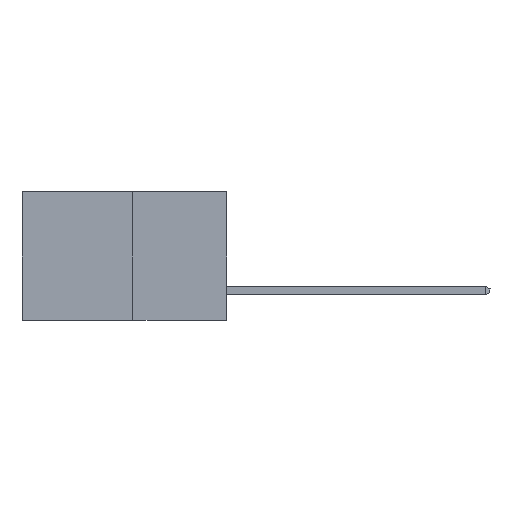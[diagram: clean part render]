
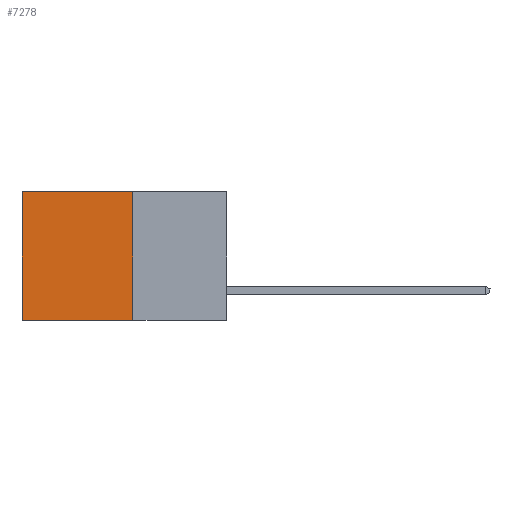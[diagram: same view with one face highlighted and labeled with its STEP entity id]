
A CAD part, left-side view. The second image highlights one B-rep face of the part: STEP entity #7278.
In plain terms, the highlighted planar face has unit normal (-1, 0, 0).
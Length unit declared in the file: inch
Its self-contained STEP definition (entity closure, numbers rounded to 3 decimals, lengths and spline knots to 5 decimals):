
#1629 = CARTESIAN_POINT ( 'NONE',  ( 0.277, 0.59, -0.37 ) ) ;
#1754 = EDGE_CURVE ( 'NONE', #6161, #5240, #4732, .T. ) ;
#4095 = VECTOR ( 'NONE', #13583, 39.37008 ) ;
#4216 = VECTOR ( 'NONE', #6669, 39.37008 ) ;
#4732 = LINE ( 'NONE', #6894, #4216 ) ;
#5116 = VERTEX_POINT ( 'NONE', #1629 ) ;
#5240 = VERTEX_POINT ( 'NONE', #7291 ) ;
#6111 = LINE ( 'NONE', #9161, #10386 ) ;
#6161 = VERTEX_POINT ( 'NONE', #14060 ) ;
#6228 = VERTEX_POINT ( 'NONE', #12454 ) ;
#6599 = DIRECTION ( 'NONE',  ( 0., 1., 0. ) ) ;
#6669 = DIRECTION ( 'NONE',  ( 0., 0., -1. ) ) ;
#6894 = CARTESIAN_POINT ( 'NONE',  ( 0.277, 0.27, -0.37 ) ) ;
#7136 = FACE_OUTER_BOUND ( 'NONE', #10306, .T. ) ;
#7278 = ADVANCED_FACE ( 'NONE', ( #7136 ), #15222, .F. ) ;
#7291 = CARTESIAN_POINT ( 'NONE',  ( 0.277, 0.27, -0.37 ) ) ;
#7445 = EDGE_CURVE ( 'NONE', #5240, #5116, #17194, .T. ) ;
#8017 = ORIENTED_EDGE ( 'NONE', *, *, #7445, .F. ) ;
#8961 = AXIS2_PLACEMENT_3D ( 'NONE', #15219, #15159, #15153 ) ;
#9161 = CARTESIAN_POINT ( 'NONE',  ( 0.277, 0.59, -0.37 ) ) ;
#9178 = VECTOR ( 'NONE', #6599, 39.37008 ) ;
#10306 = EDGE_LOOP ( 'NONE', ( #14900, #8017, #14901, #10367 ) ) ;
#10367 = ORIENTED_EDGE ( 'NONE', *, *, #18217, .T. ) ;
#10386 = VECTOR ( 'NONE', #18469, 39.37008 ) ;
#12454 = CARTESIAN_POINT ( 'NONE',  ( 0.277, 0.59, 0. ) ) ;
#13570 = CARTESIAN_POINT ( 'NONE',  ( 0.277, 0.27, -0.37 ) ) ;
#13583 = DIRECTION ( 'NONE',  ( 0., 1., 0. ) ) ;
#14060 = CARTESIAN_POINT ( 'NONE',  ( 0.277, 0.27, 0. ) ) ;
#14900 = ORIENTED_EDGE ( 'NONE', *, *, #19209, .T. ) ;
#14901 = ORIENTED_EDGE ( 'NONE', *, *, #1754, .F. ) ;
#15153 = DIRECTION ( 'NONE',  ( 0., 0., -1. ) ) ;
#15159 = DIRECTION ( 'NONE',  ( 1., 0., 0. ) ) ;
#15219 = CARTESIAN_POINT ( 'NONE',  ( 0.277, 0.27, -0.37 ) ) ;
#15222 = PLANE ( 'NONE',  #8961 ) ;
#17194 = LINE ( 'NONE', #13570, #4095 ) ;
#17468 = LINE ( 'NONE', #19056, #9178 ) ;
#18217 = EDGE_CURVE ( 'NONE', #6161, #6228, #17468, .T. ) ;
#18469 = DIRECTION ( 'NONE',  ( 0., 0., -1. ) ) ;
#19056 = CARTESIAN_POINT ( 'NONE',  ( 0.277, 0.27, 0. ) ) ;
#19209 = EDGE_CURVE ( 'NONE', #6228, #5116, #6111, .T. ) ;
